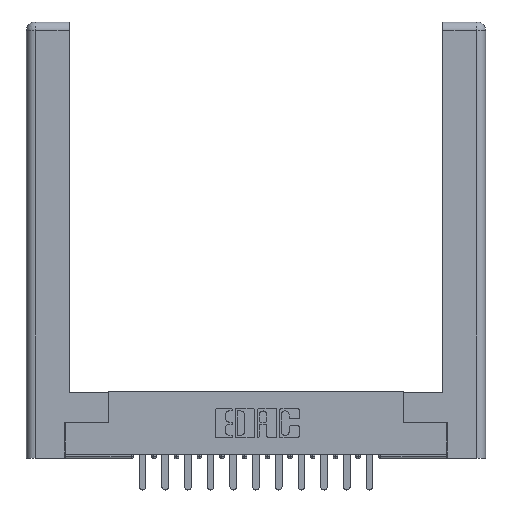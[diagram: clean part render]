
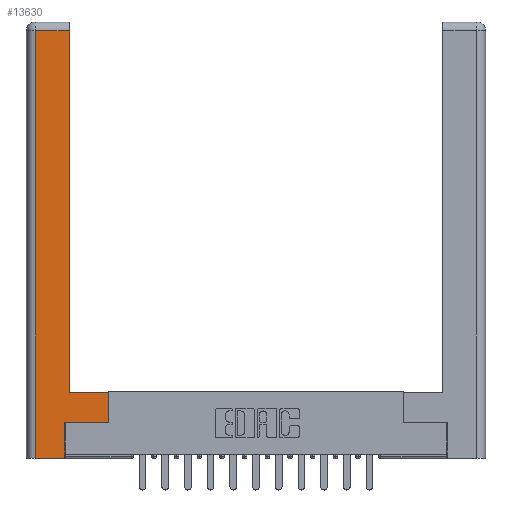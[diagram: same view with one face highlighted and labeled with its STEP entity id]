
A CAD part, top view. The second image highlights one B-rep face of the part: STEP entity #13630.
In plain terms, the highlighted planar face has unit normal (0, 0, 1).
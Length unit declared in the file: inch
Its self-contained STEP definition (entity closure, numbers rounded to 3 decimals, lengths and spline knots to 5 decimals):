
#121 = VECTOR ( 'NONE', #1536, 39.37008 ) ;
#191 = VERTEX_POINT ( 'NONE', #15067 ) ;
#242 = ORIENTED_EDGE ( 'NONE', *, *, #6703, .T. ) ;
#1536 = DIRECTION ( 'NONE',  ( -1., 0., 0. ) ) ;
#1704 = VECTOR ( 'NONE', #11512, 39.37008 ) ;
#1863 = LINE ( 'NONE', #3052, #14804 ) ;
#2113 = CARTESIAN_POINT ( 'NONE',  ( 0., 0., 0. ) ) ;
#2361 = ORIENTED_EDGE ( 'NONE', *, *, #7440, .T. ) ;
#2555 = ORIENTED_EDGE ( 'NONE', *, *, #6686, .T. ) ;
#2964 = LINE ( 'NONE', #8018, #6598 ) ;
#3052 = CARTESIAN_POINT ( 'NONE',  ( 0.265, 0., 0. ) ) ;
#3057 = AXIS2_PLACEMENT_3D ( 'NONE', #2113, #7311, #4753 ) ;
#3203 = PLANE ( 'NONE',  #3057 ) ;
#3391 = DIRECTION ( 'NONE',  ( 0., 1., 0. ) ) ;
#3422 = ORIENTED_EDGE ( 'NONE', *, *, #14744, .T. ) ;
#3622 = EDGE_LOOP ( 'NONE', ( #2361, #4864, #13580, #242, #15647, #8030, #2555, #3422 ) ) ;
#3846 = LINE ( 'NONE', #11733, #16193 ) ;
#3887 = DIRECTION ( 'NONE',  ( -1., 0., 0. ) ) ;
#4015 = DIRECTION ( 'NONE',  ( 0., 1., 0. ) ) ;
#4723 = CARTESIAN_POINT ( 'NONE',  ( 0.295, 0.45, 0. ) ) ;
#4753 = DIRECTION ( 'NONE',  ( -1., 0., 0. ) ) ;
#4864 = ORIENTED_EDGE ( 'NONE', *, *, #7859, .T. ) ;
#4981 = LINE ( 'NONE', #10034, #15399 ) ;
#4997 = VERTEX_POINT ( 'NONE', #4723 ) ;
#5308 = VERTEX_POINT ( 'NONE', #15676 ) ;
#6119 = CARTESIAN_POINT ( 'NONE',  ( 0.295, 0.45, 0. ) ) ;
#6486 = VERTEX_POINT ( 'NONE', #6665 ) ;
#6561 = LINE ( 'NONE', #10507, #121 ) ;
#6598 = VECTOR ( 'NONE', #13400, 39.37008 ) ;
#6665 = CARTESIAN_POINT ( 'NONE',  ( 0.265, 0.245, 0. ) ) ;
#6686 = EDGE_CURVE ( 'NONE', #191, #10765, #2964, .T. ) ;
#6703 = EDGE_CURVE ( 'NONE', #15071, #5308, #1863, .T. ) ;
#6746 = CARTESIAN_POINT ( 'NONE',  ( 0.295, 2.94, 0. ) ) ;
#6896 = VECTOR ( 'NONE', #3887, 39.37008 ) ;
#7311 = DIRECTION ( 'NONE',  ( 0., 0., -1. ) ) ;
#7371 = VERTEX_POINT ( 'NONE', #6746 ) ;
#7440 = EDGE_CURVE ( 'NONE', #4997, #7371, #3846, .T. ) ;
#7859 = EDGE_CURVE ( 'NONE', #7371, #10422, #6561, .T. ) ;
#8018 = CARTESIAN_POINT ( 'NONE',  ( 0.565, 0.45, 0. ) ) ;
#8030 = ORIENTED_EDGE ( 'NONE', *, *, #13710, .T. ) ;
#8270 = DIRECTION ( 'NONE',  ( 1., 0., 0. ) ) ;
#8429 = LINE ( 'NONE', #15204, #16730 ) ;
#9026 = CARTESIAN_POINT ( 'NONE',  ( 0.565, 0.245, 0. ) ) ;
#9718 = FACE_OUTER_BOUND ( 'NONE', #3622, .T. ) ;
#10034 = CARTESIAN_POINT ( 'NONE',  ( 0.0615, 0., 0. ) ) ;
#10422 = VERTEX_POINT ( 'NONE', #14034 ) ;
#10507 = CARTESIAN_POINT ( 'NONE',  ( 0.0615, 2.94, 0. ) ) ;
#10765 = VERTEX_POINT ( 'NONE', #12176 ) ;
#11512 = DIRECTION ( 'NONE',  ( 1., 0., 0. ) ) ;
#11663 = DIRECTION ( 'NONE',  ( 0., -1., 0. ) ) ;
#11733 = CARTESIAN_POINT ( 'NONE',  ( 0.295, 3., 0. ) ) ;
#12176 = CARTESIAN_POINT ( 'NONE',  ( 0.565, 0.45, 0. ) ) ;
#13400 = DIRECTION ( 'NONE',  ( 0., 1., 0. ) ) ;
#13580 = ORIENTED_EDGE ( 'NONE', *, *, #16358, .T. ) ;
#13630 = ADVANCED_FACE ( 'NONE', ( #9718 ), #3203, .F. ) ;
#13710 = EDGE_CURVE ( 'NONE', #6486, #191, #15619, .T. ) ;
#14004 = LINE ( 'NONE', #6119, #6896 ) ;
#14034 = CARTESIAN_POINT ( 'NONE',  ( 0.0615, 2.94, 0. ) ) ;
#14744 = EDGE_CURVE ( 'NONE', #10765, #4997, #14004, .T. ) ;
#14804 = VECTOR ( 'NONE', #8270, 39.37008 ) ;
#15067 = CARTESIAN_POINT ( 'NONE',  ( 0.565, 0.245, 0. ) ) ;
#15071 = VERTEX_POINT ( 'NONE', #15165 ) ;
#15165 = CARTESIAN_POINT ( 'NONE',  ( 0.0615, 0., 0. ) ) ;
#15204 = CARTESIAN_POINT ( 'NONE',  ( 0.265, 0.245, 0. ) ) ;
#15399 = VECTOR ( 'NONE', #11663, 39.37008 ) ;
#15619 = LINE ( 'NONE', #9026, #1704 ) ;
#15647 = ORIENTED_EDGE ( 'NONE', *, *, #15795, .T. ) ;
#15676 = CARTESIAN_POINT ( 'NONE',  ( 0.265, 0., 0. ) ) ;
#15795 = EDGE_CURVE ( 'NONE', #5308, #6486, #8429, .T. ) ;
#16193 = VECTOR ( 'NONE', #4015, 39.37008 ) ;
#16358 = EDGE_CURVE ( 'NONE', #10422, #15071, #4981, .T. ) ;
#16730 = VECTOR ( 'NONE', #3391, 39.37008 ) ;
